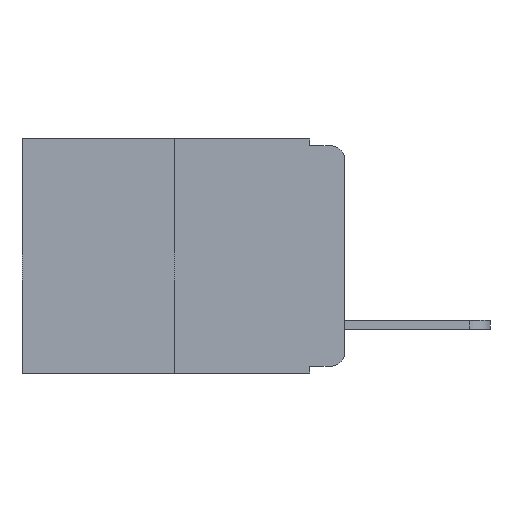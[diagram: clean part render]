
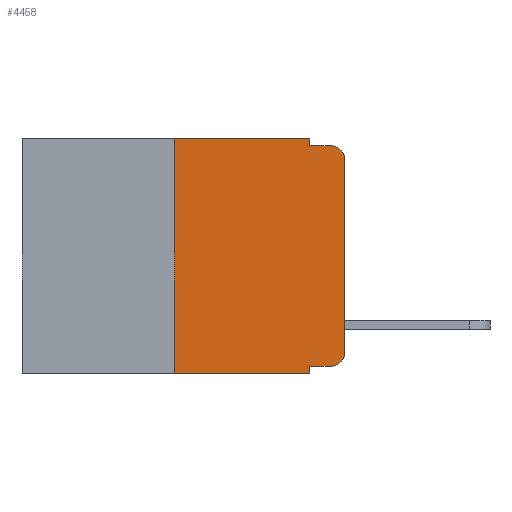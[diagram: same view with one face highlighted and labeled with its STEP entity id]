
A CAD part, left-side view. The second image highlights one B-rep face of the part: STEP entity #4458.
In plain terms, the highlighted planar face has unit normal (-1, 0, 0).
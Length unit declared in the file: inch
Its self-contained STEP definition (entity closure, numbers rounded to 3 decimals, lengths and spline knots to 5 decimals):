
#32 = ORIENTED_EDGE ( 'NONE', *, *, #1879, .F. ) ;
#287 = CARTESIAN_POINT ( 'NONE',  ( 0., 0.051, -0.343 ) ) ;
#289 = EDGE_CURVE ( 'NONE', #3655, #3896, #334, .T. ) ;
#334 = LINE ( 'NONE', #12256, #4484 ) ;
#718 = EDGE_CURVE ( 'NONE', #7310, #10958, #11687, .T. ) ;
#742 = CARTESIAN_POINT ( 'NONE',  ( 0., 0.051, -0.01 ) ) ;
#829 = DIRECTION ( 'NONE',  ( -1., 0., 0. ) ) ;
#995 = VERTEX_POINT ( 'NONE', #287 ) ;
#1081 = CARTESIAN_POINT ( 'NONE',  ( 0., 0.02, -0.03 ) ) ;
#1086 = AXIS2_PLACEMENT_3D ( 'NONE', #11090, #829, #3583 ) ;
#1205 = DIRECTION ( 'NONE',  ( 0., 0., -1. ) ) ;
#1243 = CARTESIAN_POINT ( 'NONE',  ( 0., 0.051, -0.333 ) ) ;
#1791 = DIRECTION ( 'NONE',  ( 0., 0., -1. ) ) ;
#1879 = EDGE_CURVE ( 'NONE', #10958, #9998, #8025, .T. ) ;
#2090 = VECTOR ( 'NONE', #4357, 39.37008 ) ;
#2103 = LINE ( 'NONE', #9955, #5831 ) ;
#2186 = DIRECTION ( 'NONE',  ( 0., -1., 0. ) ) ;
#2309 = VECTOR ( 'NONE', #10136, 39.37008 ) ;
#2991 = CARTESIAN_POINT ( 'NONE',  ( 0., 0.25, -0.343 ) ) ;
#3129 = DIRECTION ( 'NONE',  ( -1., 0., 0. ) ) ;
#3245 = EDGE_CURVE ( 'NONE', #3655, #995, #7448, .T. ) ;
#3275 = ORIENTED_EDGE ( 'NONE', *, *, #289, .T. ) ;
#3353 = ORIENTED_EDGE ( 'NONE', *, *, #718, .F. ) ;
#3456 = AXIS2_PLACEMENT_3D ( 'NONE', #10301, #9309, #1791 ) ;
#3583 = DIRECTION ( 'NONE',  ( 0., 0., -1. ) ) ;
#3655 = VERTEX_POINT ( 'NONE', #1243 ) ;
#3677 = ORIENTED_EDGE ( 'NONE', *, *, #7928, .T. ) ;
#3896 = VERTEX_POINT ( 'NONE', #5752 ) ;
#4136 = ORIENTED_EDGE ( 'NONE', *, *, #7203, .T. ) ;
#4319 = EDGE_LOOP ( 'NONE', ( #3677, #7513, #5814, #8527, #32, #3353, #4136, #9852, #3275, #9830 ) ) ;
#4357 = DIRECTION ( 'NONE',  ( 0., 0., -1. ) ) ;
#4458 = ADVANCED_FACE ( 'NONE', ( #10834 ), #6479, .F. ) ;
#4461 = VECTOR ( 'NONE', #2186, 39.37008 ) ;
#4484 = VECTOR ( 'NONE', #6938, 39.37008 ) ;
#5124 = CARTESIAN_POINT ( 'NONE',  ( 0., 0.051, 0. ) ) ;
#5219 = EDGE_CURVE ( 'NONE', #3896, #9999, #8482, .T. ) ;
#5274 = CARTESIAN_POINT ( 'NONE',  ( 0., 0.051, 0. ) ) ;
#5620 = CARTESIAN_POINT ( 'NONE',  ( 0., 0.051, -0.01 ) ) ;
#5640 = DIRECTION ( 'NONE',  ( 0., 0., 1. ) ) ;
#5644 = VECTOR ( 'NONE', #12184, 39.37008 ) ;
#5752 = CARTESIAN_POINT ( 'NONE',  ( 0., 0.02, -0.333 ) ) ;
#5814 = ORIENTED_EDGE ( 'NONE', *, *, #11952, .F. ) ;
#5831 = VECTOR ( 'NONE', #10901, 39.37008 ) ;
#5917 = CARTESIAN_POINT ( 'NONE',  ( 0., 0.473, -0.343 ) ) ;
#5963 = VERTEX_POINT ( 'NONE', #5620 ) ;
#6122 = EDGE_CURVE ( 'NONE', #6552, #6668, #6841, .T. ) ;
#6406 = VECTOR ( 'NONE', #5640, 39.37008 ) ;
#6479 = PLANE ( 'NONE',  #3456 ) ;
#6552 = VERTEX_POINT ( 'NONE', #10195 ) ;
#6668 = VERTEX_POINT ( 'NONE', #9618 ) ;
#6841 = CIRCLE ( 'NONE', #9480, 0.02 ) ;
#6938 = DIRECTION ( 'NONE',  ( 0., -1., 0. ) ) ;
#7203 = EDGE_CURVE ( 'NONE', #7310, #995, #7633, .T. ) ;
#7310 = VERTEX_POINT ( 'NONE', #2991 ) ;
#7332 = VECTOR ( 'NONE', #10631, 39.37008 ) ;
#7448 = LINE ( 'NONE', #5274, #2090 ) ;
#7513 = ORIENTED_EDGE ( 'NONE', *, *, #6122, .T. ) ;
#7633 = LINE ( 'NONE', #5917, #7332 ) ;
#7701 = LINE ( 'NONE', #10277, #5644 ) ;
#7928 = EDGE_CURVE ( 'NONE', #9999, #6552, #2103, .T. ) ;
#7987 = CARTESIAN_POINT ( 'NONE',  ( 0., 0., -0.313 ) ) ;
#8025 = LINE ( 'NONE', #8685, #4461 ) ;
#8223 = CARTESIAN_POINT ( 'NONE',  ( 0., 0.25, 0. ) ) ;
#8482 = CIRCLE ( 'NONE', #1086, 0.02 ) ;
#8527 = ORIENTED_EDGE ( 'NONE', *, *, #10211, .F. ) ;
#8685 = CARTESIAN_POINT ( 'NONE',  ( 0., 0.473, 0. ) ) ;
#8827 = LINE ( 'NONE', #742, #2309 ) ;
#9309 = DIRECTION ( 'NONE',  ( 1., 0., 0. ) ) ;
#9360 = CARTESIAN_POINT ( 'NONE',  ( 0., 0.25, 0. ) ) ;
#9480 = AXIS2_PLACEMENT_3D ( 'NONE', #1081, #3129, #1205 ) ;
#9618 = CARTESIAN_POINT ( 'NONE',  ( 0., 0.02, -0.01 ) ) ;
#9830 = ORIENTED_EDGE ( 'NONE', *, *, #5219, .T. ) ;
#9852 = ORIENTED_EDGE ( 'NONE', *, *, #3245, .F. ) ;
#9955 = CARTESIAN_POINT ( 'NONE',  ( 0., 0., 0. ) ) ;
#9998 = VERTEX_POINT ( 'NONE', #5124 ) ;
#9999 = VERTEX_POINT ( 'NONE', #7987 ) ;
#10136 = DIRECTION ( 'NONE',  ( 0., -1., 0. ) ) ;
#10195 = CARTESIAN_POINT ( 'NONE',  ( 0., 0., -0.03 ) ) ;
#10211 = EDGE_CURVE ( 'NONE', #9998, #5963, #7701, .T. ) ;
#10277 = CARTESIAN_POINT ( 'NONE',  ( 0., 0.051, 0. ) ) ;
#10301 = CARTESIAN_POINT ( 'NONE',  ( 0., 0.473, 0. ) ) ;
#10631 = DIRECTION ( 'NONE',  ( 0., -1., 0. ) ) ;
#10834 = FACE_OUTER_BOUND ( 'NONE', #4319, .T. ) ;
#10901 = DIRECTION ( 'NONE',  ( 0., 0., 1. ) ) ;
#10958 = VERTEX_POINT ( 'NONE', #9360 ) ;
#11090 = CARTESIAN_POINT ( 'NONE',  ( 0., 0.02, -0.313 ) ) ;
#11687 = LINE ( 'NONE', #8223, #6406 ) ;
#11952 = EDGE_CURVE ( 'NONE', #5963, #6668, #8827, .T. ) ;
#12184 = DIRECTION ( 'NONE',  ( 0., 0., -1. ) ) ;
#12256 = CARTESIAN_POINT ( 'NONE',  ( 0., 0.051, -0.333 ) ) ;
